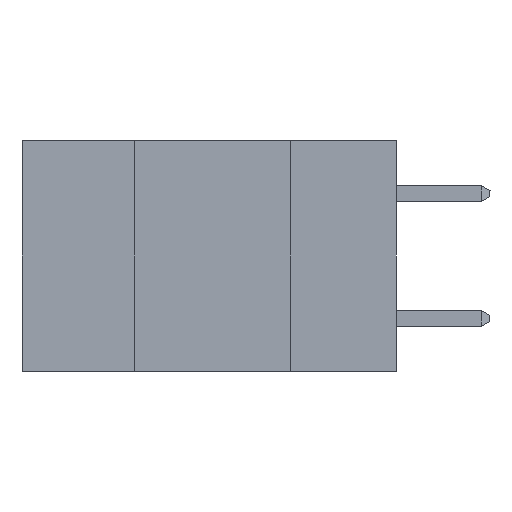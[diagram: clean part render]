
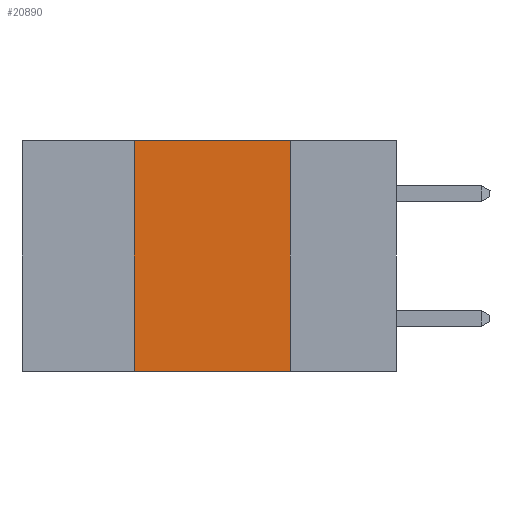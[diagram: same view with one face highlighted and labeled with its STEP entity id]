
A CAD part, left-side view. The second image highlights one B-rep face of the part: STEP entity #20890.
In plain terms, the highlighted planar face has unit normal (-1, 0, 0).
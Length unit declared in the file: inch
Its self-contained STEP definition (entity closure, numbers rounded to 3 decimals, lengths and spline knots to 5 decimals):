
#14 = VERTEX_POINT ( 'NONE', #2844 ) ;
#813 = CARTESIAN_POINT ( 'NONE',  ( 0., 0.6, 0. ) ) ;
#1640 = FACE_OUTER_BOUND ( 'NONE', #5999, .T. ) ;
#1930 = DIRECTION ( 'NONE',  ( 0., 0., -1. ) ) ;
#2369 = CARTESIAN_POINT ( 'NONE',  ( 0., 0.42, 0. ) ) ;
#2697 = DIRECTION ( 'NONE',  ( 0., 0., -1. ) ) ;
#2844 = CARTESIAN_POINT ( 'NONE',  ( 0., 0.17, 0. ) ) ;
#2853 = DIRECTION ( 'NONE',  ( 1., 0., 0. ) ) ;
#3272 = VERTEX_POINT ( 'NONE', #23854 ) ;
#3960 = VECTOR ( 'NONE', #9471, 39.37008 ) ;
#3978 = ORIENTED_EDGE ( 'NONE', *, *, #20207, .F. ) ;
#4235 = ORIENTED_EDGE ( 'NONE', *, *, #9009, .F. ) ;
#4259 = LINE ( 'NONE', #11347, #3960 ) ;
#4406 = CARTESIAN_POINT ( 'NONE',  ( 0., 0.6, -0.37 ) ) ;
#4877 = VECTOR ( 'NONE', #8101, 39.37008 ) ;
#5000 = VERTEX_POINT ( 'NONE', #17754 ) ;
#5402 = ORIENTED_EDGE ( 'NONE', *, *, #21684, .T. ) ;
#5610 = CARTESIAN_POINT ( 'NONE',  ( 0., 0.17, 0. ) ) ;
#5795 = VECTOR ( 'NONE', #12616, 39.37008 ) ;
#5999 = EDGE_LOOP ( 'NONE', ( #4235, #20526, #3978, #5402 ) ) ;
#8101 = DIRECTION ( 'NONE',  ( 0., -1., 0. ) ) ;
#9009 = EDGE_CURVE ( 'NONE', #14, #3272, #17228, .T. ) ;
#9471 = DIRECTION ( 'NONE',  ( 0., -1., 0. ) ) ;
#9813 = LINE ( 'NONE', #4406, #4877 ) ;
#10953 = CARTESIAN_POINT ( 'NONE',  ( 0., 0.42, 0. ) ) ;
#11347 = CARTESIAN_POINT ( 'NONE',  ( 0., 0.6, 0. ) ) ;
#11759 = VERTEX_POINT ( 'NONE', #2369 ) ;
#11916 = VECTOR ( 'NONE', #1930, 39.37008 ) ;
#12616 = DIRECTION ( 'NONE',  ( 0., 0., 1. ) ) ;
#15021 = EDGE_CURVE ( 'NONE', #11759, #14, #4259, .T. ) ;
#17228 = LINE ( 'NONE', #5610, #11916 ) ;
#17754 = CARTESIAN_POINT ( 'NONE',  ( 0., 0.42, -0.37 ) ) ;
#19679 = PLANE ( 'NONE',  #23889 ) ;
#20207 = EDGE_CURVE ( 'NONE', #5000, #11759, #20990, .T. ) ;
#20526 = ORIENTED_EDGE ( 'NONE', *, *, #15021, .F. ) ;
#20890 = ADVANCED_FACE ( 'NONE', ( #1640 ), #19679, .F. ) ;
#20990 = LINE ( 'NONE', #10953, #5795 ) ;
#21684 = EDGE_CURVE ( 'NONE', #5000, #3272, #9813, .T. ) ;
#23854 = CARTESIAN_POINT ( 'NONE',  ( 0., 0.17, -0.37 ) ) ;
#23889 = AXIS2_PLACEMENT_3D ( 'NONE', #813, #2853, #2697 ) ;
